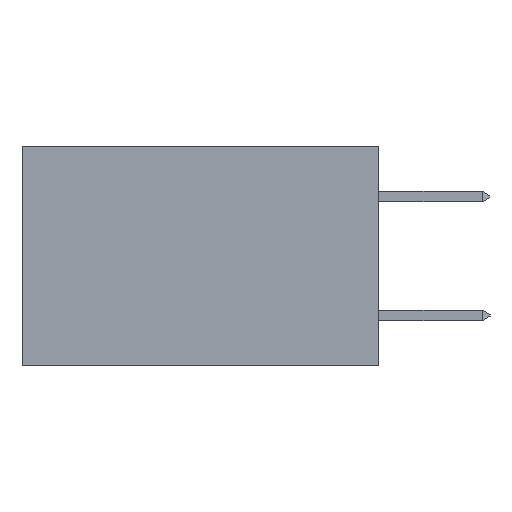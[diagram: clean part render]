
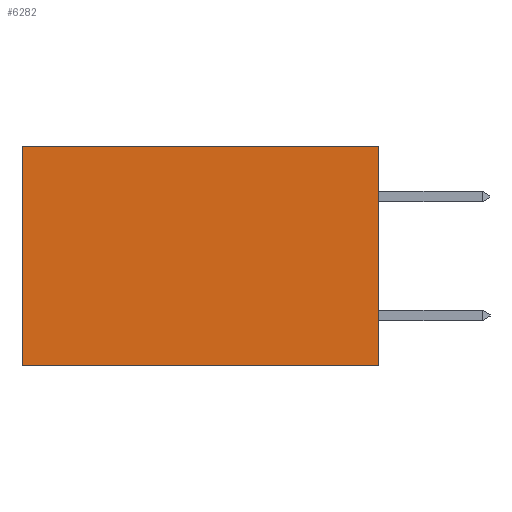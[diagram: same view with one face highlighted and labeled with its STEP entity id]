
A CAD part, left-side view. The second image highlights one B-rep face of the part: STEP entity #6282.
In plain terms, the highlighted planar face has unit normal (-1, 0, 0).
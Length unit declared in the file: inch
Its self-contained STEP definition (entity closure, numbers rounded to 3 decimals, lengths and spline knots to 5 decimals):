
#225 = ORIENTED_EDGE ( 'NONE', *, *, #6065, .T. ) ;
#295 = DIRECTION ( 'NONE',  ( 0., 1., 0. ) ) ;
#387 = CARTESIAN_POINT ( 'NONE',  ( 0.2615, 0.6, -0.37 ) ) ;
#596 = VECTOR ( 'NONE', #9170, 39.37008 ) ;
#1140 = CARTESIAN_POINT ( 'NONE',  ( 0.2615, 0., -0.37 ) ) ;
#1265 = CARTESIAN_POINT ( 'NONE',  ( 0.2615, 0., -0.37 ) ) ;
#1430 = EDGE_CURVE ( 'NONE', #10193, #5811, #9372, .T. ) ;
#3221 = FACE_OUTER_BOUND ( 'NONE', #4680, .T. ) ;
#3373 = VECTOR ( 'NONE', #10977, 39.37008 ) ;
#4680 = EDGE_LOOP ( 'NONE', ( #225, #5031, #5112, #6863 ) ) ;
#5023 = CARTESIAN_POINT ( 'NONE',  ( 0.2615, 0.6, -0.37 ) ) ;
#5031 = ORIENTED_EDGE ( 'NONE', *, *, #1430, .F. ) ;
#5112 = ORIENTED_EDGE ( 'NONE', *, *, #6542, .F. ) ;
#5800 = DIRECTION ( 'NONE',  ( 0., 0., -1. ) ) ;
#5811 = VERTEX_POINT ( 'NONE', #5023 ) ;
#5818 = PLANE ( 'NONE',  #6924 ) ;
#5835 = LINE ( 'NONE', #387, #596 ) ;
#5871 = DIRECTION ( 'NONE',  ( 1., 0., 0. ) ) ;
#6065 = EDGE_CURVE ( 'NONE', #7788, #5811, #5835, .T. ) ;
#6282 = ADVANCED_FACE ( 'NONE', ( #3221 ), #5818, .F. ) ;
#6452 = CARTESIAN_POINT ( 'NONE',  ( 0.2615, 0., 0. ) ) ;
#6498 = EDGE_CURVE ( 'NONE', #7624, #7788, #10620, .T. ) ;
#6521 = CARTESIAN_POINT ( 'NONE',  ( 0.2615, 0., -0.37 ) ) ;
#6542 = EDGE_CURVE ( 'NONE', #7624, #10193, #9587, .T. ) ;
#6863 = ORIENTED_EDGE ( 'NONE', *, *, #6498, .T. ) ;
#6924 = AXIS2_PLACEMENT_3D ( 'NONE', #6521, #5871, #5800 ) ;
#7480 = CARTESIAN_POINT ( 'NONE',  ( 0.2615, 0.6, 0. ) ) ;
#7624 = VERTEX_POINT ( 'NONE', #6452 ) ;
#7788 = VERTEX_POINT ( 'NONE', #7480 ) ;
#9097 = VECTOR ( 'NONE', #295, 39.37008 ) ;
#9170 = DIRECTION ( 'NONE',  ( 0., 0., -1. ) ) ;
#9372 = LINE ( 'NONE', #1140, #9097 ) ;
#9530 = VECTOR ( 'NONE', #10163, 39.37008 ) ;
#9587 = LINE ( 'NONE', #10196, #9530 ) ;
#10163 = DIRECTION ( 'NONE',  ( 0., 0., -1. ) ) ;
#10193 = VERTEX_POINT ( 'NONE', #1265 ) ;
#10196 = CARTESIAN_POINT ( 'NONE',  ( 0.2615, 0., -0.37 ) ) ;
#10620 = LINE ( 'NONE', #10803, #3373 ) ;
#10803 = CARTESIAN_POINT ( 'NONE',  ( 0.2615, 0., 0. ) ) ;
#10977 = DIRECTION ( 'NONE',  ( 0., 1., 0. ) ) ;
